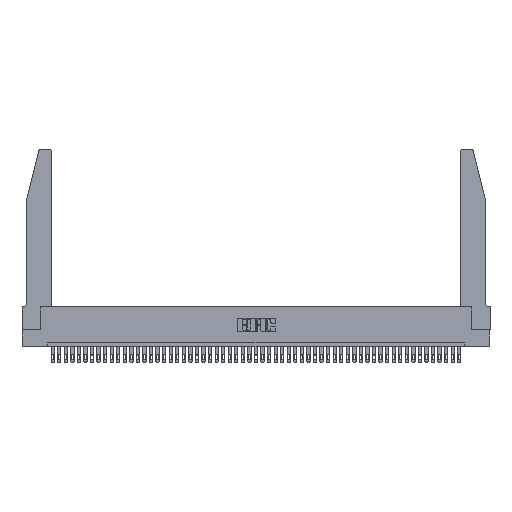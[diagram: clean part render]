
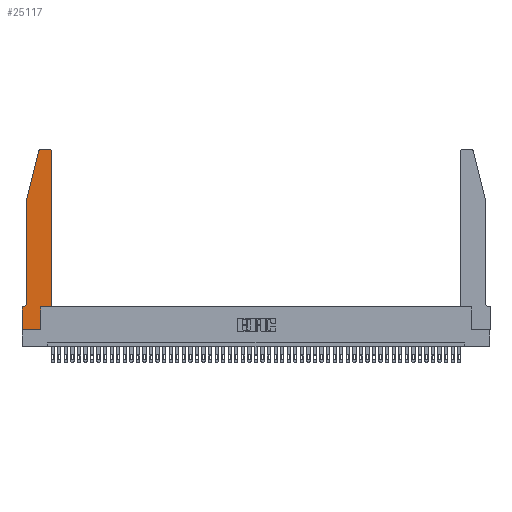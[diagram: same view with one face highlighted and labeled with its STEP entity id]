
A CAD part, top view. The second image highlights one B-rep face of the part: STEP entity #25117.
In plain terms, the highlighted planar face has unit normal (0, 0, 1).
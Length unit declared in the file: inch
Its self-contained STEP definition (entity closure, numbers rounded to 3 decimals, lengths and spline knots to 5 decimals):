
#348 = AXIS2_PLACEMENT_3D ( 'NONE', #648, #7668, #19152 ) ;
#487 = VECTOR ( 'NONE', #15197, 39.37008 ) ;
#643 = EDGE_CURVE ( 'NONE', #36702, #41289, #41600, .T. ) ;
#648 = CARTESIAN_POINT ( 'NONE',  ( 0.4205, 2.72, 0.37 ) ) ;
#1032 = ORIENTED_EDGE ( 'NONE', *, *, #643, .T. ) ;
#1149 = VERTEX_POINT ( 'NONE', #11309 ) ;
#1206 = EDGE_CURVE ( 'NONE', #27987, #29627, #14132, .T. ) ;
#1307 = VECTOR ( 'NONE', #31410, 39.37008 ) ;
#1506 = CARTESIAN_POINT ( 'NONE',  ( 0.2605, 2.75, 0.37 ) ) ;
#3357 = CARTESIAN_POINT ( 'NONE',  ( 0.4205, 2.75, 0.37 ) ) ;
#4079 = EDGE_CURVE ( 'NONE', #4255, #26333, #31866, .T. ) ;
#4255 = VERTEX_POINT ( 'NONE', #25084 ) ;
#4730 = CARTESIAN_POINT ( 'NONE',  ( 0., 0., 0.37 ) ) ;
#4865 = CARTESIAN_POINT ( 'NONE',  ( 0.0755, 0.42, 0.37 ) ) ;
#4887 = DIRECTION ( 'NONE',  ( -1., 0., 0. ) ) ;
#6034 = ORIENTED_EDGE ( 'NONE', *, *, #47748, .T. ) ;
#7668 = DIRECTION ( 'NONE',  ( 0., 0., 1. ) ) ;
#9117 = VECTOR ( 'NONE', #11851, 39.37008 ) ;
#9200 = ORIENTED_EDGE ( 'NONE', *, *, #14741, .T. ) ;
#10328 = DIRECTION ( 'NONE',  ( 1., 0., 0. ) ) ;
#10910 = CIRCLE ( 'NONE', #348, 0.03 ) ;
#11309 = CARTESIAN_POINT ( 'NONE',  ( 0.0055, 0.35, 0.37 ) ) ;
#11340 = PLANE ( 'NONE',  #26508 ) ;
#11551 = DIRECTION ( 'NONE',  ( -1., 0., 0. ) ) ;
#11851 = DIRECTION ( 'NONE',  ( 0., 1., 0. ) ) ;
#13126 = LINE ( 'NONE', #1506, #48941 ) ;
#14132 = LINE ( 'NONE', #29642, #31985 ) ;
#14741 = EDGE_CURVE ( 'NONE', #41289, #46831, #17951, .T. ) ;
#15197 = DIRECTION ( 'NONE',  ( 1., 0., 0. ) ) ;
#16228 = DIRECTION ( 'NONE',  ( 0., -1., 0. ) ) ;
#16391 = CARTESIAN_POINT ( 'NONE',  ( 0.0755, 2., 0.37 ) ) ;
#17000 = CARTESIAN_POINT ( 'NONE',  ( 0.4505, 2.72, 0.37 ) ) ;
#17951 = LINE ( 'NONE', #29937, #37021 ) ;
#18042 = LINE ( 'NONE', #16391, #35890 ) ;
#18629 = DIRECTION ( 'NONE',  ( 1., 0., 0. ) ) ;
#18713 = VERTEX_POINT ( 'NONE', #3357 ) ;
#19152 = DIRECTION ( 'NONE',  ( 1., 0., 0. ) ) ;
#19670 = DIRECTION ( 'NONE',  ( 0., 0., -1. ) ) ;
#20406 = EDGE_CURVE ( 'NONE', #1149, #27987, #45789, .T. ) ;
#21706 = VERTEX_POINT ( 'NONE', #4865 ) ;
#22046 = CARTESIAN_POINT ( 'NONE',  ( 0.284, 2.72, 0.37 ) ) ;
#23630 = EDGE_CURVE ( 'NONE', #28966, #18713, #10910, .T. ) ;
#23900 = ORIENTED_EDGE ( 'NONE', *, *, #4079, .T. ) ;
#24430 = ORIENTED_EDGE ( 'NONE', *, *, #23630, .T. ) ;
#24769 = EDGE_CURVE ( 'NONE', #35962, #21706, #18042, .T. ) ;
#24966 = VECTOR ( 'NONE', #4887, 39.37008 ) ;
#25084 = CARTESIAN_POINT ( 'NONE',  ( 0.284, 2.75, 0.37 ) ) ;
#25117 = ADVANCED_FACE ( 'NONE', ( #47808 ), #11340, .T. ) ;
#25560 = CARTESIAN_POINT ( 'NONE',  ( 0.0755, 2., 0.37 ) ) ;
#25711 = ORIENTED_EDGE ( 'NONE', *, *, #44149, .T. ) ;
#26333 = VERTEX_POINT ( 'NONE', #43566 ) ;
#26508 = AXIS2_PLACEMENT_3D ( 'NONE', #27758, #33486, #10328 ) ;
#26813 = CARTESIAN_POINT ( 'NONE',  ( 0.4505, 0.35, 0.37 ) ) ;
#27758 = CARTESIAN_POINT ( 'NONE',  ( 0., 0.35, 0.37 ) ) ;
#27987 = VERTEX_POINT ( 'NONE', #42832 ) ;
#28632 = ORIENTED_EDGE ( 'NONE', *, *, #24769, .T. ) ;
#28966 = VERTEX_POINT ( 'NONE', #17000 ) ;
#29627 = VERTEX_POINT ( 'NONE', #4730 ) ;
#29642 = CARTESIAN_POINT ( 'NONE',  ( 0., 0., 0.37 ) ) ;
#29901 = ORIENTED_EDGE ( 'NONE', *, *, #20406, .T. ) ;
#29937 = CARTESIAN_POINT ( 'NONE',  ( 0.4505, 0.35, 0.37 ) ) ;
#30024 = DIRECTION ( 'NONE',  ( 1., 0., 0. ) ) ;
#30241 = EDGE_CURVE ( 'NONE', #26333, #35962, #35235, .T. ) ;
#31084 = EDGE_CURVE ( 'NONE', #21706, #1149, #32221, .T. ) ;
#31410 = DIRECTION ( 'NONE',  ( -0.239, -0.971, 0. ) ) ;
#31866 = CIRCLE ( 'NONE', #34536, 0.03 ) ;
#31985 = VECTOR ( 'NONE', #36836, 39.37008 ) ;
#32221 = CIRCLE ( 'NONE', #34962, 0.07 ) ;
#32666 = DIRECTION ( 'NONE',  ( 0., 1., 0. ) ) ;
#32770 = LINE ( 'NONE', #34650, #487 ) ;
#33486 = DIRECTION ( 'NONE',  ( 0., 0., 1. ) ) ;
#34536 = AXIS2_PLACEMENT_3D ( 'NONE', #22046, #49213, #30024 ) ;
#34650 = CARTESIAN_POINT ( 'NONE',  ( 0., 0., 0.37 ) ) ;
#34962 = AXIS2_PLACEMENT_3D ( 'NONE', #38362, #19670, #11551 ) ;
#35235 = LINE ( 'NONE', #35277, #1307 ) ;
#35277 = CARTESIAN_POINT ( 'NONE',  ( 0.0755, 2., 0.37 ) ) ;
#35325 = CARTESIAN_POINT ( 'NONE',  ( 0.0755, 0.35, 0.37 ) ) ;
#35890 = VECTOR ( 'NONE', #16228, 39.37008 ) ;
#35962 = VERTEX_POINT ( 'NONE', #25560 ) ;
#36650 = CARTESIAN_POINT ( 'NONE',  ( 0.2865, 0.35, 0.37 ) ) ;
#36702 = VERTEX_POINT ( 'NONE', #48146 ) ;
#36744 = ORIENTED_EDGE ( 'NONE', *, *, #1206, .T. ) ;
#36836 = DIRECTION ( 'NONE',  ( 0., -1., 0. ) ) ;
#37021 = VECTOR ( 'NONE', #18629, 39.37008 ) ;
#38173 = ORIENTED_EDGE ( 'NONE', *, *, #46247, .T. ) ;
#38362 = CARTESIAN_POINT ( 'NONE',  ( 0.0055, 0.42, 0.37 ) ) ;
#38674 = ORIENTED_EDGE ( 'NONE', *, *, #30241, .T. ) ;
#38686 = CARTESIAN_POINT ( 'NONE',  ( 0.4505, 0.35, 0.37 ) ) ;
#39255 = CARTESIAN_POINT ( 'NONE',  ( 0.2865, 0.35, 0.37 ) ) ;
#40256 = EDGE_LOOP ( 'NONE', ( #6034, #23900, #38674, #28632, #44691, #29901, #36744, #25711, #1032, #9200, #38173, #24430 ) ) ;
#41289 = VERTEX_POINT ( 'NONE', #36650 ) ;
#41600 = LINE ( 'NONE', #39255, #43411 ) ;
#42832 = CARTESIAN_POINT ( 'NONE',  ( 0., 0.35, 0.37 ) ) ;
#43411 = VECTOR ( 'NONE', #32666, 39.37008 ) ;
#43438 = DIRECTION ( 'NONE',  ( -1., 0., 0. ) ) ;
#43566 = CARTESIAN_POINT ( 'NONE',  ( 0.25487, 2.72718, 0.37 ) ) ;
#44149 = EDGE_CURVE ( 'NONE', #29627, #36702, #32770, .T. ) ;
#44691 = ORIENTED_EDGE ( 'NONE', *, *, #31084, .T. ) ;
#45520 = LINE ( 'NONE', #38686, #9117 ) ;
#45789 = LINE ( 'NONE', #35325, #24966 ) ;
#46247 = EDGE_CURVE ( 'NONE', #46831, #28966, #45520, .T. ) ;
#46831 = VERTEX_POINT ( 'NONE', #26813 ) ;
#47748 = EDGE_CURVE ( 'NONE', #18713, #4255, #13126, .T. ) ;
#47808 = FACE_OUTER_BOUND ( 'NONE', #40256, .T. ) ;
#48146 = CARTESIAN_POINT ( 'NONE',  ( 0.2865, 0., 0.37 ) ) ;
#48941 = VECTOR ( 'NONE', #43438, 39.37008 ) ;
#49213 = DIRECTION ( 'NONE',  ( 0., 0., 1. ) ) ;
